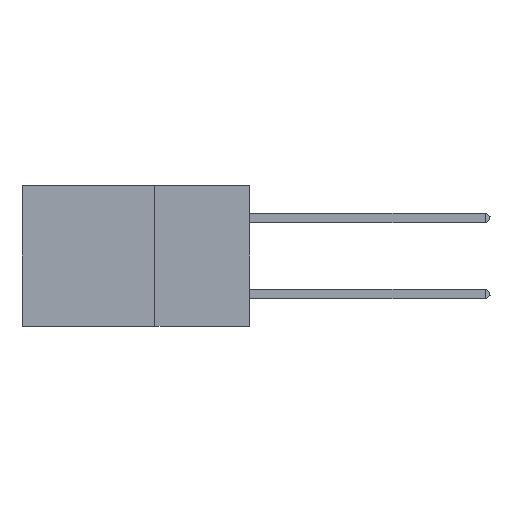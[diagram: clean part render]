
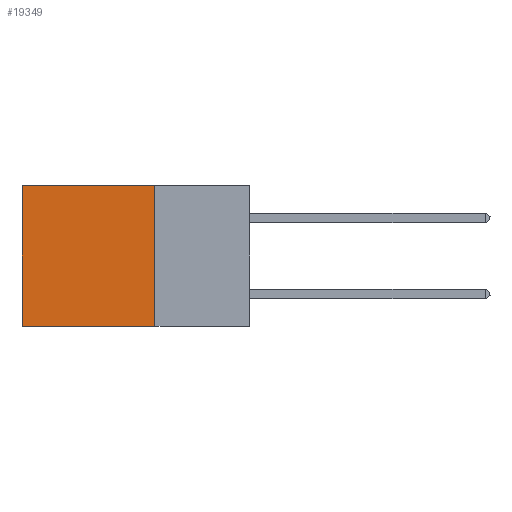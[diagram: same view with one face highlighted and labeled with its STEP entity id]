
A CAD part, left-side view. The second image highlights one B-rep face of the part: STEP entity #19349.
In plain terms, the highlighted planar face has unit normal (-1, 0, 0).
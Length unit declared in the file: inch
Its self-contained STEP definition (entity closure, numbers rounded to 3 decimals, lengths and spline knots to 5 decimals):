
#265 = VECTOR ( 'NONE', #7444, 39.37008 ) ;
#1318 = LINE ( 'NONE', #19970, #9453 ) ;
#2420 = EDGE_LOOP ( 'NONE', ( #3654, #4696, #14157, #16713 ) ) ;
#2468 = CARTESIAN_POINT ( 'NONE',  ( 0.2875, 0.6, 0. ) ) ;
#2526 = VERTEX_POINT ( 'NONE', #12292 ) ;
#3382 = DIRECTION ( 'NONE',  ( 0., 0., -1. ) ) ;
#3654 = ORIENTED_EDGE ( 'NONE', *, *, #5060, .T. ) ;
#4167 = PLANE ( 'NONE',  #7204 ) ;
#4696 = ORIENTED_EDGE ( 'NONE', *, *, #7733, .F. ) ;
#5060 = EDGE_CURVE ( 'NONE', #19036, #9871, #6466, .T. ) ;
#5578 = LINE ( 'NONE', #11590, #6123 ) ;
#5692 = CARTESIAN_POINT ( 'NONE',  ( 0.2875, 0.25, -0.37 ) ) ;
#5948 = DIRECTION ( 'NONE',  ( 1., 0., 0. ) ) ;
#6123 = VECTOR ( 'NONE', #21389, 39.37008 ) ;
#6223 = CARTESIAN_POINT ( 'NONE',  ( 0.2875, 0.6, -0.37 ) ) ;
#6466 = LINE ( 'NONE', #6935, #15420 ) ;
#6935 = CARTESIAN_POINT ( 'NONE',  ( 0.2875, 0.6, 0. ) ) ;
#7204 = AXIS2_PLACEMENT_3D ( 'NONE', #16014, #5948, #17674 ) ;
#7353 = EDGE_CURVE ( 'NONE', #2526, #19036, #5578, .T. ) ;
#7444 = DIRECTION ( 'NONE',  ( 0., 1., 0. ) ) ;
#7733 = EDGE_CURVE ( 'NONE', #8654, #9871, #17314, .T. ) ;
#8654 = VERTEX_POINT ( 'NONE', #11326 ) ;
#9078 = FACE_OUTER_BOUND ( 'NONE', #2420, .T. ) ;
#9453 = VECTOR ( 'NONE', #3382, 39.37008 ) ;
#9871 = VERTEX_POINT ( 'NONE', #6223 ) ;
#11326 = CARTESIAN_POINT ( 'NONE',  ( 0.2875, 0.25, -0.37 ) ) ;
#11590 = CARTESIAN_POINT ( 'NONE',  ( 0.2875, 0.25, 0. ) ) ;
#12292 = CARTESIAN_POINT ( 'NONE',  ( 0.2875, 0.25, 0. ) ) ;
#14157 = ORIENTED_EDGE ( 'NONE', *, *, #20322, .F. ) ;
#15420 = VECTOR ( 'NONE', #18604, 39.37008 ) ;
#16014 = CARTESIAN_POINT ( 'NONE',  ( 0.2875, 0.25, 0. ) ) ;
#16713 = ORIENTED_EDGE ( 'NONE', *, *, #7353, .T. ) ;
#17314 = LINE ( 'NONE', #5692, #265 ) ;
#17674 = DIRECTION ( 'NONE',  ( 0., 0., -1. ) ) ;
#18604 = DIRECTION ( 'NONE',  ( 0., 0., -1. ) ) ;
#19036 = VERTEX_POINT ( 'NONE', #2468 ) ;
#19349 = ADVANCED_FACE ( 'NONE', ( #9078 ), #4167, .F. ) ;
#19970 = CARTESIAN_POINT ( 'NONE',  ( 0.2875, 0.25, 0. ) ) ;
#20322 = EDGE_CURVE ( 'NONE', #2526, #8654, #1318, .T. ) ;
#21389 = DIRECTION ( 'NONE',  ( 0., 1., 0. ) ) ;
